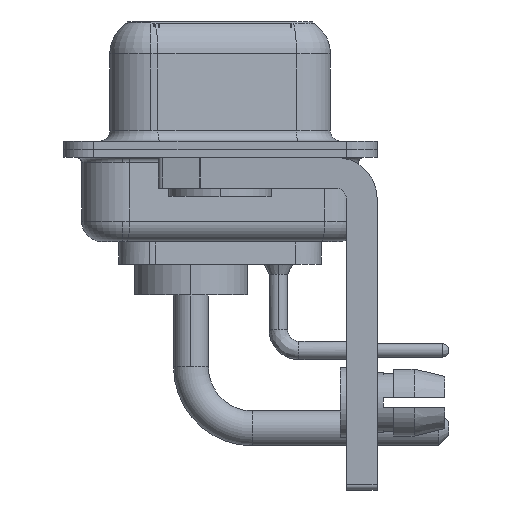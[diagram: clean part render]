
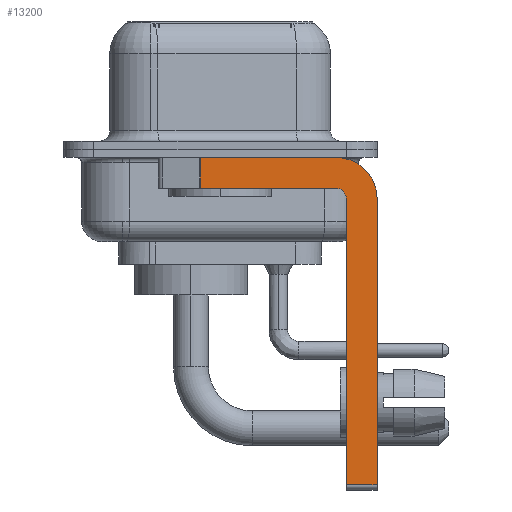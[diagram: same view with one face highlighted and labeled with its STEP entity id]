
A CAD part, left-side view. The second image highlights one B-rep face of the part: STEP entity #13200.
In plain terms, the highlighted planar face has unit normal (-1, 0, 0).
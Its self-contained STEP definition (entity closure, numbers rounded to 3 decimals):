
#1057 = CARTESIAN_POINT ( 'NONE',  ( -2.9, -7.65, -16.35 ) ) ;
#1100 = CARTESIAN_POINT ( 'NONE',  ( -2.9, -7.65, -2.4 ) ) ;
#1161 = DIRECTION ( 'NONE',  ( -1., 0., 0. ) ) ;
#1196 = ORIENTED_EDGE ( 'NONE', *, *, #22738, .F. ) ;
#1398 = DIRECTION ( 'NONE',  ( 0., -1., 0. ) ) ;
#1564 = DIRECTION ( 'NONE',  ( 0., 0., 1. ) ) ;
#2073 = VECTOR ( 'NONE', #11803, 1000. ) ;
#2761 = CARTESIAN_POINT ( 'NONE',  ( -2.9, 0.978, -1.9 ) ) ;
#3072 = DIRECTION ( 'NONE',  ( 0., 0., 1. ) ) ;
#3531 = FACE_OUTER_BOUND ( 'NONE', #8741, .T. ) ;
#4156 = ORIENTED_EDGE ( 'NONE', *, *, #6082, .F. ) ;
#4891 = CARTESIAN_POINT ( 'NONE',  ( -2.9, -5.65, -2.4 ) ) ;
#4916 = CIRCLE ( 'NONE', #7186, 2. ) ;
#5010 = LINE ( 'NONE', #21247, #10213 ) ;
#5023 = EDGE_CURVE ( 'NONE', #6613, #5647, #17798, .T. ) ;
#5389 = CARTESIAN_POINT ( 'NONE',  ( -2.9, -7.65, -2.4 ) ) ;
#5460 = DIRECTION ( 'NONE',  ( 1., 0., 0. ) ) ;
#5500 = VERTEX_POINT ( 'NONE', #7769 ) ;
#5647 = VERTEX_POINT ( 'NONE', #7400 ) ;
#5709 = VECTOR ( 'NONE', #1564, 1000. ) ;
#5727 = ORIENTED_EDGE ( 'NONE', *, *, #10252, .F. ) ;
#6082 = EDGE_CURVE ( 'NONE', #6941, #15529, #8566, .T. ) ;
#6496 = DIRECTION ( 'NONE',  ( 0., 0., -1. ) ) ;
#6613 = VERTEX_POINT ( 'NONE', #9336 ) ;
#6718 = DIRECTION ( 'NONE',  ( 0., 0., -1. ) ) ;
#6941 = VERTEX_POINT ( 'NONE', #21498 ) ;
#7173 = ORIENTED_EDGE ( 'NONE', *, *, #16903, .T. ) ;
#7186 = AXIS2_PLACEMENT_3D ( 'NONE', #22934, #17664, #6718 ) ;
#7400 = CARTESIAN_POINT ( 'NONE',  ( -2.9, -6.15, -2.4 ) ) ;
#7613 = VERTEX_POINT ( 'NONE', #13047 ) ;
#7769 = CARTESIAN_POINT ( 'NONE',  ( -2.9, -5.65, -0.4 ) ) ;
#7964 = ORIENTED_EDGE ( 'NONE', *, *, #22094, .F. ) ;
#8212 = CARTESIAN_POINT ( 'NONE',  ( -2.9, -5.65, -1.9 ) ) ;
#8337 = CARTESIAN_POINT ( 'NONE',  ( -2.9, 0.978, -1.9 ) ) ;
#8566 = LINE ( 'NONE', #8212, #16783 ) ;
#8741 = EDGE_LOOP ( 'NONE', ( #7964, #20153, #4156, #21281, #12579, #7173, #5727, #1196 ) ) ;
#9336 = CARTESIAN_POINT ( 'NONE',  ( -2.9, -6.15, -16.35 ) ) ;
#10057 = LINE ( 'NONE', #1100, #13449 ) ;
#10213 = VECTOR ( 'NONE', #1398, 1000. ) ;
#10252 = EDGE_CURVE ( 'NONE', #15735, #14195, #10057, .T. ) ;
#11250 = AXIS2_PLACEMENT_3D ( 'NONE', #17954, #5460, #19998 ) ;
#11803 = DIRECTION ( 'NONE',  ( 0., 0., -1. ) ) ;
#12562 = EDGE_CURVE ( 'NONE', #5647, #6941, #15096, .T. ) ;
#12579 = ORIENTED_EDGE ( 'NONE', *, *, #5023, .F. ) ;
#13047 = CARTESIAN_POINT ( 'NONE',  ( -2.9, 0.978, -0.4 ) ) ;
#13200 = ADVANCED_FACE ( 'NONE', ( #3531 ), #23341, .F. ) ;
#13449 = VECTOR ( 'NONE', #6496, 1000. ) ;
#13740 = LINE ( 'NONE', #15545, #16905 ) ;
#14195 = VERTEX_POINT ( 'NONE', #1057 ) ;
#15096 = CIRCLE ( 'NONE', #19663, 0.5 ) ;
#15257 = LINE ( 'NONE', #8337, #2073 ) ;
#15529 = VERTEX_POINT ( 'NONE', #2761 ) ;
#15545 = CARTESIAN_POINT ( 'NONE',  ( -2.9, -5.65, -16.35 ) ) ;
#15735 = VERTEX_POINT ( 'NONE', #5389 ) ;
#16783 = VECTOR ( 'NONE', #21121, 1000. ) ;
#16903 = EDGE_CURVE ( 'NONE', #6613, #14195, #13740, .T. ) ;
#16905 = VECTOR ( 'NONE', #20941, 1000. ) ;
#17664 = DIRECTION ( 'NONE',  ( 1., 0., 0. ) ) ;
#17798 = LINE ( 'NONE', #21296, #5709 ) ;
#17954 = CARTESIAN_POINT ( 'NONE',  ( -2.9, -5.65, -2.4 ) ) ;
#19203 = EDGE_CURVE ( 'NONE', #7613, #15529, #15257, .T. ) ;
#19663 = AXIS2_PLACEMENT_3D ( 'NONE', #4891, #1161, #3072 ) ;
#19998 = DIRECTION ( 'NONE',  ( 0., 0., -1. ) ) ;
#20153 = ORIENTED_EDGE ( 'NONE', *, *, #19203, .T. ) ;
#20941 = DIRECTION ( 'NONE',  ( 0., -1., 0. ) ) ;
#21121 = DIRECTION ( 'NONE',  ( 0., 1., 0. ) ) ;
#21247 = CARTESIAN_POINT ( 'NONE',  ( -2.9, 3., -0.4 ) ) ;
#21281 = ORIENTED_EDGE ( 'NONE', *, *, #12562, .F. ) ;
#21296 = CARTESIAN_POINT ( 'NONE',  ( -2.9, -6.15, -16.6 ) ) ;
#21498 = CARTESIAN_POINT ( 'NONE',  ( -2.9, -5.65, -1.9 ) ) ;
#22094 = EDGE_CURVE ( 'NONE', #7613, #5500, #5010, .T. ) ;
#22738 = EDGE_CURVE ( 'NONE', #5500, #15735, #4916, .T. ) ;
#22934 = CARTESIAN_POINT ( 'NONE',  ( -2.9, -5.65, -2.4 ) ) ;
#23341 = PLANE ( 'NONE',  #11250 ) ;
